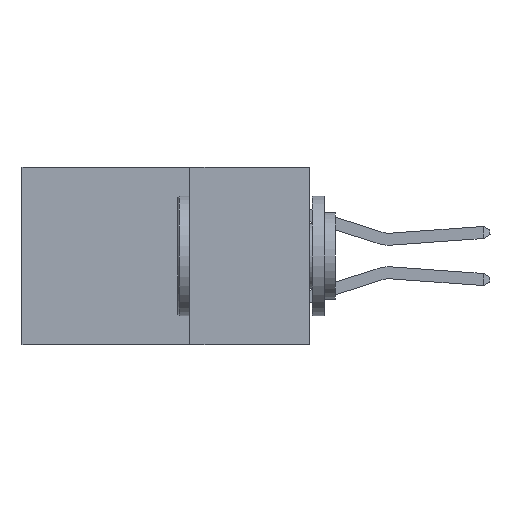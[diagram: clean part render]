
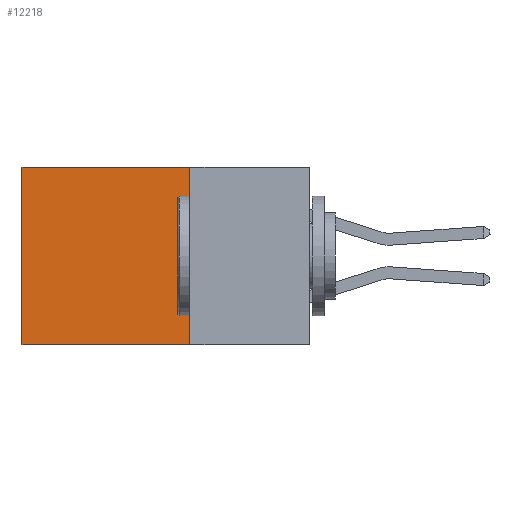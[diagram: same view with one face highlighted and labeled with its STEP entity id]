
A CAD part, left-side view. The second image highlights one B-rep face of the part: STEP entity #12218.
In plain terms, the highlighted planar face has unit normal (-1, 0, 0).
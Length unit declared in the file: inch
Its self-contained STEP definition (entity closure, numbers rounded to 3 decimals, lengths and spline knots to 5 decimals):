
#279 = VERTEX_POINT ( 'NONE', #3439 ) ;
#506 = EDGE_CURVE ( 'NONE', #9355, #5020, #4001, .T. ) ;
#567 = ORIENTED_EDGE ( 'NONE', *, *, #3474, .F. ) ;
#832 = CARTESIAN_POINT ( 'NONE',  ( 0.298, 0.25, 0. ) ) ;
#2543 = ORIENTED_EDGE ( 'NONE', *, *, #506, .F. ) ;
#2603 = DIRECTION ( 'NONE',  ( 0., 0., -1. ) ) ;
#2748 = EDGE_LOOP ( 'NONE', ( #7841, #2543, #567, #7302 ) ) ;
#2823 = CARTESIAN_POINT ( 'NONE',  ( 0.298, 0.25, -0.37 ) ) ;
#3293 = DIRECTION ( 'NONE',  ( 0., 0., -1. ) ) ;
#3439 = CARTESIAN_POINT ( 'NONE',  ( 0.298, 0.6, 0. ) ) ;
#3474 = EDGE_CURVE ( 'NONE', #9284, #9355, #11526, .T. ) ;
#3803 = DIRECTION ( 'NONE',  ( 0., 1., 0. ) ) ;
#4001 = LINE ( 'NONE', #2823, #11171 ) ;
#4232 = LINE ( 'NONE', #9305, #11999 ) ;
#4302 = EDGE_CURVE ( 'NONE', #279, #5020, #10891, .T. ) ;
#4306 = PLANE ( 'NONE',  #7945 ) ;
#4526 = CARTESIAN_POINT ( 'NONE',  ( 0.298, 0.6, 0. ) ) ;
#5020 = VERTEX_POINT ( 'NONE', #8415 ) ;
#5368 = DIRECTION ( 'NONE',  ( 0., 1., 0. ) ) ;
#6980 = CARTESIAN_POINT ( 'NONE',  ( 0.298, 0.25, 0. ) ) ;
#7179 = CARTESIAN_POINT ( 'NONE',  ( 0.298, 0.25, 0. ) ) ;
#7302 = ORIENTED_EDGE ( 'NONE', *, *, #11215, .T. ) ;
#7676 = VECTOR ( 'NONE', #2603, 39.37008 ) ;
#7841 = ORIENTED_EDGE ( 'NONE', *, *, #4302, .T. ) ;
#7945 = AXIS2_PLACEMENT_3D ( 'NONE', #7179, #12188, #3293 ) ;
#8276 = CARTESIAN_POINT ( 'NONE',  ( 0.298, 0.25, -0.37 ) ) ;
#8415 = CARTESIAN_POINT ( 'NONE',  ( 0.298, 0.6, -0.37 ) ) ;
#9284 = VERTEX_POINT ( 'NONE', #6980 ) ;
#9305 = CARTESIAN_POINT ( 'NONE',  ( 0.298, 0.25, 0. ) ) ;
#9355 = VERTEX_POINT ( 'NONE', #8276 ) ;
#9539 = VECTOR ( 'NONE', #9619, 39.37008 ) ;
#9619 = DIRECTION ( 'NONE',  ( 0., 0., -1. ) ) ;
#9839 = FACE_OUTER_BOUND ( 'NONE', #2748, .T. ) ;
#10891 = LINE ( 'NONE', #4526, #7676 ) ;
#11171 = VECTOR ( 'NONE', #3803, 39.37008 ) ;
#11215 = EDGE_CURVE ( 'NONE', #9284, #279, #4232, .T. ) ;
#11526 = LINE ( 'NONE', #832, #9539 ) ;
#11999 = VECTOR ( 'NONE', #5368, 39.37008 ) ;
#12188 = DIRECTION ( 'NONE',  ( 1., 0., 0. ) ) ;
#12218 = ADVANCED_FACE ( 'NONE', ( #9839 ), #4306, .F. ) ;
